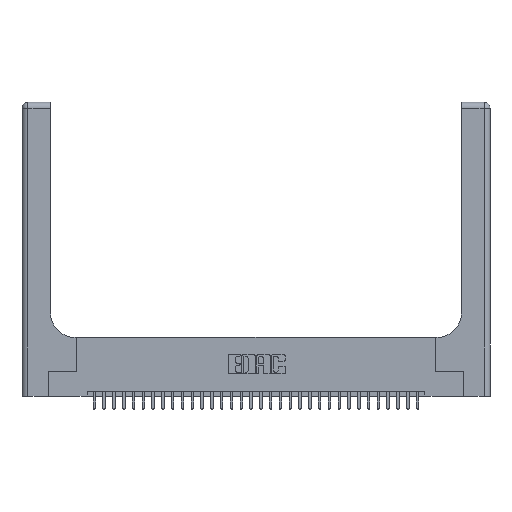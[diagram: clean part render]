
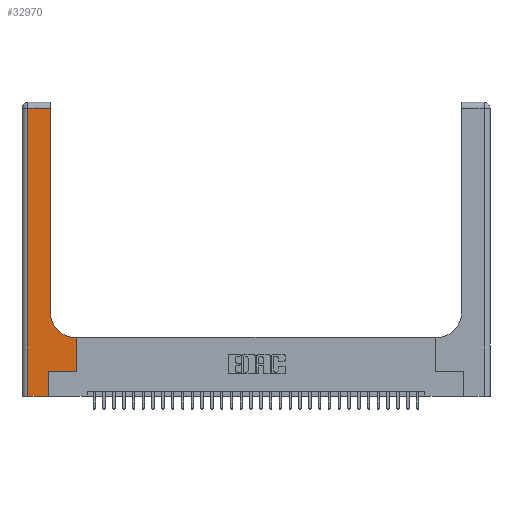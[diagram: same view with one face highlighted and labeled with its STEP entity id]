
A CAD part, top view. The second image highlights one B-rep face of the part: STEP entity #32970.
In plain terms, the highlighted planar face has unit normal (0, 0, 1).
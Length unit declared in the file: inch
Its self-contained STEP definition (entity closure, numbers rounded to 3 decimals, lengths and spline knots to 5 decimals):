
#105 = DIRECTION ( 'NONE',  ( -1., 0., 0. ) ) ;
#429 = CARTESIAN_POINT ( 'NONE',  ( 0.269, 0., 0.37 ) ) ;
#452 = ORIENTED_EDGE ( 'NONE', *, *, #26867, .T. ) ;
#540 = CARTESIAN_POINT ( 'NONE',  ( 0.2915, 0.6, 0.37 ) ) ;
#1142 = LINE ( 'NONE', #26231, #12329 ) ;
#1222 = CARTESIAN_POINT ( 'NONE',  ( 0.06, 2.94, 0.37 ) ) ;
#1370 = DIRECTION ( 'NONE',  ( 1., 0., 0. ) ) ;
#1682 = VECTOR ( 'NONE', #12430, 39.37008 ) ;
#2427 = FACE_OUTER_BOUND ( 'NONE', #8736, .T. ) ;
#2575 = ORIENTED_EDGE ( 'NONE', *, *, #16709, .T. ) ;
#2664 = DIRECTION ( 'NONE',  ( 0., 0., -1. ) ) ;
#3388 = EDGE_CURVE ( 'NONE', #4355, #13769, #28142, .T. ) ;
#3673 = VERTEX_POINT ( 'NONE', #21536 ) ;
#3886 = VECTOR ( 'NONE', #9611, 39.37008 ) ;
#3917 = CARTESIAN_POINT ( 'NONE',  ( 0.5415, 0.6, 0.37 ) ) ;
#4099 = VERTEX_POINT ( 'NONE', #32474 ) ;
#4355 = VERTEX_POINT ( 'NONE', #19324 ) ;
#4358 = ORIENTED_EDGE ( 'NONE', *, *, #3388, .T. ) ;
#5581 = EDGE_CURVE ( 'NONE', #29507, #4355, #1142, .T. ) ;
#6201 = VECTOR ( 'NONE', #15229, 39.37008 ) ;
#6680 = EDGE_CURVE ( 'NONE', #11716, #4099, #14983, .T. ) ;
#6872 = LINE ( 'NONE', #32233, #1682 ) ;
#7015 = LINE ( 'NONE', #30411, #6201 ) ;
#7321 = EDGE_CURVE ( 'NONE', #3673, #27370, #7015, .T. ) ;
#7483 = VECTOR ( 'NONE', #22307, 39.37008 ) ;
#8568 = AXIS2_PLACEMENT_3D ( 'NONE', #20516, #29666, #1370 ) ;
#8736 = EDGE_LOOP ( 'NONE', ( #13684, #452, #23238, #32648, #2575, #29009, #4358, #13549, #22141 ) ) ;
#9383 = LINE ( 'NONE', #540, #14531 ) ;
#9611 = DIRECTION ( 'NONE',  ( 0., 1., 0. ) ) ;
#9911 = CARTESIAN_POINT ( 'NONE',  ( 0.269, 0., 0.37 ) ) ;
#10707 = DIRECTION ( 'NONE',  ( -1., 0., 0. ) ) ;
#11508 = CARTESIAN_POINT ( 'NONE',  ( 0.269, 0.25, 0.37 ) ) ;
#11716 = VERTEX_POINT ( 'NONE', #3917 ) ;
#12329 = VECTOR ( 'NONE', #19297, 39.37008 ) ;
#12430 = DIRECTION ( 'NONE',  ( 0., 1., 0. ) ) ;
#12577 = LINE ( 'NONE', #31391, #13340 ) ;
#12904 = EDGE_CURVE ( 'NONE', #19661, #3673, #13226, .T. ) ;
#13226 = LINE ( 'NONE', #13574, #20361 ) ;
#13340 = VECTOR ( 'NONE', #23388, 39.37008 ) ;
#13435 = EDGE_CURVE ( 'NONE', #4099, #21486, #6872, .T. ) ;
#13549 = ORIENTED_EDGE ( 'NONE', *, *, #20351, .T. ) ;
#13574 = CARTESIAN_POINT ( 'NONE',  ( 0.06, 3., 0.37 ) ) ;
#13684 = ORIENTED_EDGE ( 'NONE', *, *, #13435, .T. ) ;
#13769 = VERTEX_POINT ( 'NONE', #25824 ) ;
#14531 = VECTOR ( 'NONE', #10707, 39.37008 ) ;
#14983 = CIRCLE ( 'NONE', #8568, 0.25 ) ;
#15229 = DIRECTION ( 'NONE',  ( 1., 0., 0. ) ) ;
#15368 = LINE ( 'NONE', #9911, #7483 ) ;
#16709 = EDGE_CURVE ( 'NONE', #27370, #29507, #15368, .T. ) ;
#18375 = DIRECTION ( 'NONE',  ( 0., -1., 0. ) ) ;
#19297 = DIRECTION ( 'NONE',  ( 1., 0., 0. ) ) ;
#19324 = CARTESIAN_POINT ( 'NONE',  ( 0.5585, 0.25, 0.37 ) ) ;
#19661 = VERTEX_POINT ( 'NONE', #1222 ) ;
#20321 = PLANE ( 'NONE',  #24345 ) ;
#20351 = EDGE_CURVE ( 'NONE', #13769, #11716, #9383, .T. ) ;
#20361 = VECTOR ( 'NONE', #18375, 39.37008 ) ;
#20516 = CARTESIAN_POINT ( 'NONE',  ( 0.5415, 0.85, 0.37 ) ) ;
#21486 = VERTEX_POINT ( 'NONE', #21712 ) ;
#21536 = CARTESIAN_POINT ( 'NONE',  ( 0.06, 0., 0.37 ) ) ;
#21712 = CARTESIAN_POINT ( 'NONE',  ( 0.2915, 2.94, 0.37 ) ) ;
#22141 = ORIENTED_EDGE ( 'NONE', *, *, #6680, .T. ) ;
#22307 = DIRECTION ( 'NONE',  ( 0., 1., 0. ) ) ;
#23238 = ORIENTED_EDGE ( 'NONE', *, *, #12904, .T. ) ;
#23388 = DIRECTION ( 'NONE',  ( -1., 0., 0. ) ) ;
#24345 = AXIS2_PLACEMENT_3D ( 'NONE', #30632, #2664, #105 ) ;
#25824 = CARTESIAN_POINT ( 'NONE',  ( 0.5585, 0.6, 0.37 ) ) ;
#26231 = CARTESIAN_POINT ( 'NONE',  ( 0.269, 0.25, 0.37 ) ) ;
#26867 = EDGE_CURVE ( 'NONE', #21486, #19661, #12577, .T. ) ;
#27370 = VERTEX_POINT ( 'NONE', #429 ) ;
#27516 = CARTESIAN_POINT ( 'NONE',  ( 0.5585, 0.25, 0.37 ) ) ;
#28142 = LINE ( 'NONE', #27516, #3886 ) ;
#29009 = ORIENTED_EDGE ( 'NONE', *, *, #5581, .T. ) ;
#29507 = VERTEX_POINT ( 'NONE', #11508 ) ;
#29666 = DIRECTION ( 'NONE',  ( 0., 0., -1. ) ) ;
#30411 = CARTESIAN_POINT ( 'NONE',  ( 0., 0., 0.37 ) ) ;
#30632 = CARTESIAN_POINT ( 'NONE',  ( 0., 3., 0.37 ) ) ;
#31391 = CARTESIAN_POINT ( 'NONE',  ( 0., 2.94, 0.37 ) ) ;
#32233 = CARTESIAN_POINT ( 'NONE',  ( 0.2915, 3., 0.37 ) ) ;
#32474 = CARTESIAN_POINT ( 'NONE',  ( 0.2915, 0.85, 0.37 ) ) ;
#32648 = ORIENTED_EDGE ( 'NONE', *, *, #7321, .T. ) ;
#32970 = ADVANCED_FACE ( 'NONE', ( #2427 ), #20321, .F. ) ;
